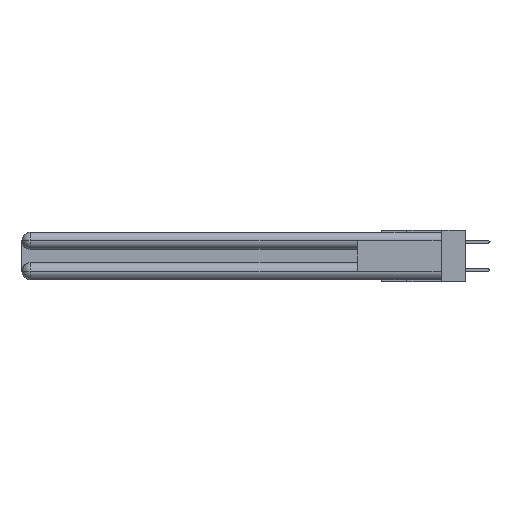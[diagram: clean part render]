
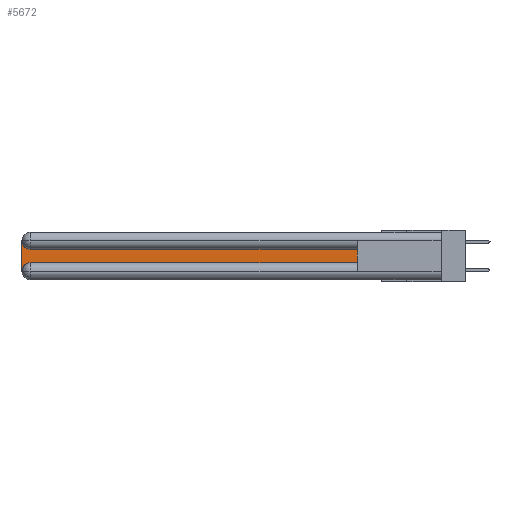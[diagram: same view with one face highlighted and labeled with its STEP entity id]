
A CAD part, left-side view. The second image highlights one B-rep face of the part: STEP entity #5672.
In plain terms, the highlighted planar face has unit normal (-1, 0, 0).
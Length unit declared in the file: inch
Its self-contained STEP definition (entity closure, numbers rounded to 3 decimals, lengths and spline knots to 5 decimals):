
#180 = CARTESIAN_POINT ( 'NONE',  ( 0.075, 2.94, -0.1225 ) ) ;
#1046 = DIRECTION ( 'NONE',  ( 1., 0., 0. ) ) ;
#1778 = EDGE_CURVE ( 'NONE', #3647, #19659, #22241, .T. ) ;
#2056 = ORIENTED_EDGE ( 'NONE', *, *, #15110, .T. ) ;
#2260 = DIRECTION ( 'NONE',  ( 0., 1., 0. ) ) ;
#2318 = EDGE_CURVE ( 'NONE', #22162, #3725, #2432, .T. ) ;
#2432 = LINE ( 'NONE', #26062, #32241 ) ;
#3069 = EDGE_CURVE ( 'NONE', #23498, #22162, #15499, .T. ) ;
#3647 = VERTEX_POINT ( 'NONE', #6325 ) ;
#3725 = VERTEX_POINT ( 'NONE', #14704 ) ;
#4169 = CARTESIAN_POINT ( 'NONE',  ( 0.075, 0.6, -0.1225 ) ) ;
#4870 = EDGE_CURVE ( 'NONE', #19659, #23498, #6306, .T. ) ;
#5672 = ADVANCED_FACE ( 'NONE', ( #22362 ), #6172, .F. ) ;
#6172 = PLANE ( 'NONE',  #26129 ) ;
#6306 = CIRCLE ( 'NONE', #20500, 0.06 ) ;
#6325 = CARTESIAN_POINT ( 'NONE',  ( 0.075, 3., -0.0625 ) ) ;
#6492 = VECTOR ( 'NONE', #14257, 39.37008 ) ;
#6661 = CARTESIAN_POINT ( 'NONE',  ( 0.075, 2.94, -0.2175 ) ) ;
#7471 = CARTESIAN_POINT ( 'NONE',  ( 0.075, 3., -0.2775 ) ) ;
#8372 = CARTESIAN_POINT ( 'NONE',  ( 0.075, 3., -0.1225 ) ) ;
#11864 = CARTESIAN_POINT ( 'NONE',  ( 0.075, 0.6, -0.2175 ) ) ;
#13283 = VERTEX_POINT ( 'NONE', #180 ) ;
#13284 = VECTOR ( 'NONE', #2260, 39.37008 ) ;
#14257 = DIRECTION ( 'NONE',  ( 0., 0., -1. ) ) ;
#14704 = CARTESIAN_POINT ( 'NONE',  ( 0.075, 0.6, -0.1225 ) ) ;
#15110 = EDGE_CURVE ( 'NONE', #3725, #13283, #19947, .T. ) ;
#15499 = LINE ( 'NONE', #11864, #30650 ) ;
#15947 = CARTESIAN_POINT ( 'NONE',  ( 0.075, 2.94, -0.2775 ) ) ;
#17817 = ORIENTED_EDGE ( 'NONE', *, *, #22926, .T. ) ;
#18033 = ORIENTED_EDGE ( 'NONE', *, *, #4870, .T. ) ;
#18699 = DIRECTION ( 'NONE',  ( 0., 0., -1. ) ) ;
#19659 = VERTEX_POINT ( 'NONE', #7471 ) ;
#19947 = LINE ( 'NONE', #4169, #13284 ) ;
#20500 = AXIS2_PLACEMENT_3D ( 'NONE', #15947, #26398, #26181 ) ;
#21227 = DIRECTION ( 'NONE',  ( 1., 0., 0. ) ) ;
#21858 = DIRECTION ( 'NONE',  ( 0., -1., 0. ) ) ;
#22075 = ORIENTED_EDGE ( 'NONE', *, *, #1778, .T. ) ;
#22162 = VERTEX_POINT ( 'NONE', #24146 ) ;
#22241 = LINE ( 'NONE', #32025, #6492 ) ;
#22362 = FACE_OUTER_BOUND ( 'NONE', #31752, .T. ) ;
#22926 = EDGE_CURVE ( 'NONE', #13283, #3647, #26450, .T. ) ;
#23498 = VERTEX_POINT ( 'NONE', #6661 ) ;
#23834 = DIRECTION ( 'NONE',  ( 0., 0., -1. ) ) ;
#24146 = CARTESIAN_POINT ( 'NONE',  ( 0.075, 0.6, -0.2175 ) ) ;
#26062 = CARTESIAN_POINT ( 'NONE',  ( 0.075, 0.6, -0.2175 ) ) ;
#26074 = ORIENTED_EDGE ( 'NONE', *, *, #3069, .T. ) ;
#26129 = AXIS2_PLACEMENT_3D ( 'NONE', #8372, #1046, #18699 ) ;
#26181 = DIRECTION ( 'NONE',  ( 0., 0., -1. ) ) ;
#26398 = DIRECTION ( 'NONE',  ( 1., 0., 0. ) ) ;
#26450 = CIRCLE ( 'NONE', #28777, 0.06 ) ;
#28777 = AXIS2_PLACEMENT_3D ( 'NONE', #31420, #21227, #23834 ) ;
#30650 = VECTOR ( 'NONE', #21858, 39.37008 ) ;
#31167 = ORIENTED_EDGE ( 'NONE', *, *, #2318, .T. ) ;
#31420 = CARTESIAN_POINT ( 'NONE',  ( 0.075, 2.94, -0.0625 ) ) ;
#31609 = DIRECTION ( 'NONE',  ( 0., 0., 1. ) ) ;
#31752 = EDGE_LOOP ( 'NONE', ( #2056, #17817, #22075, #18033, #26074, #31167 ) ) ;
#32025 = CARTESIAN_POINT ( 'NONE',  ( 0.075, 3., -0.2175 ) ) ;
#32241 = VECTOR ( 'NONE', #31609, 39.37008 ) ;
